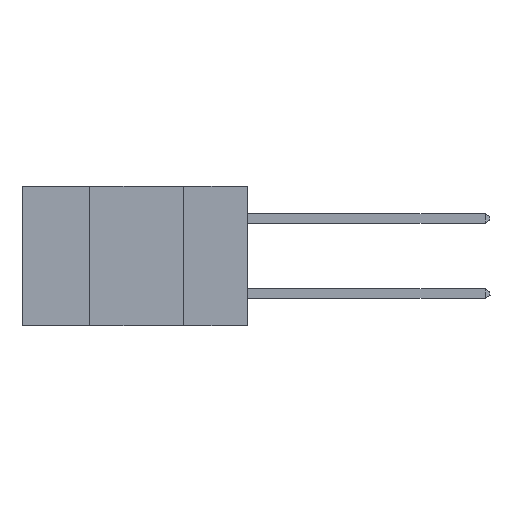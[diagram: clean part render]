
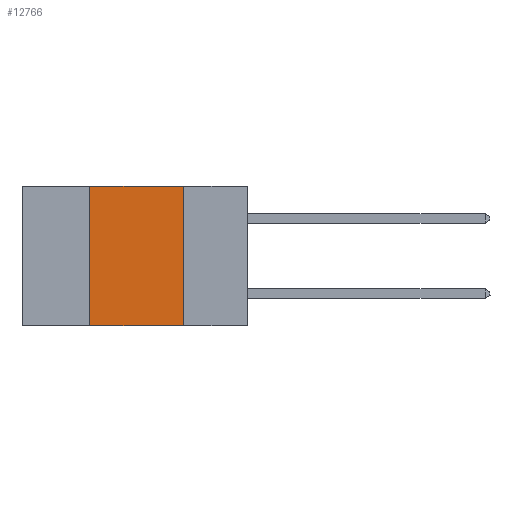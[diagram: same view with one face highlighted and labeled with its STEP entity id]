
A CAD part, left-side view. The second image highlights one B-rep face of the part: STEP entity #12766.
In plain terms, the highlighted planar face has unit normal (-1, 0, 0).
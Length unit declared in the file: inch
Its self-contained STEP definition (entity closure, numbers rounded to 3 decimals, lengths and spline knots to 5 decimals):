
#288 = EDGE_CURVE ( 'NONE', #16798, #23068, #29079, .T. ) ;
#878 = LINE ( 'NONE', #9492, #11123 ) ;
#1423 = CARTESIAN_POINT ( 'NONE',  ( 0., 0.42, 0. ) ) ;
#1833 = DIRECTION ( 'NONE',  ( 0., 0., -1. ) ) ;
#1933 = DIRECTION ( 'NONE',  ( 1., 0., 0. ) ) ;
#2817 = VECTOR ( 'NONE', #6527, 39.37008 ) ;
#5611 = DIRECTION ( 'NONE',  ( 0., -1., 0. ) ) ;
#6152 = VECTOR ( 'NONE', #5611, 39.37008 ) ;
#6527 = DIRECTION ( 'NONE',  ( 0., -1., 0. ) ) ;
#8866 = CARTESIAN_POINT ( 'NONE',  ( 0., 0.6, 0. ) ) ;
#8895 = EDGE_CURVE ( 'NONE', #28290, #23068, #17753, .T. ) ;
#9492 = CARTESIAN_POINT ( 'NONE',  ( 0., 0.42, 0. ) ) ;
#11123 = VECTOR ( 'NONE', #16550, 39.37008 ) ;
#11801 = ORIENTED_EDGE ( 'NONE', *, *, #12406, .F. ) ;
#12406 = EDGE_CURVE ( 'NONE', #28290, #13880, #878, .T. ) ;
#12438 = EDGE_CURVE ( 'NONE', #13880, #16798, #18273, .T. ) ;
#12471 = CARTESIAN_POINT ( 'NONE',  ( 0., 0.6, 0. ) ) ;
#12766 = ADVANCED_FACE ( 'NONE', ( #17528 ), #22303, .F. ) ;
#13751 = CARTESIAN_POINT ( 'NONE',  ( 0., 0.17, 0. ) ) ;
#13880 = VERTEX_POINT ( 'NONE', #1423 ) ;
#14284 = CARTESIAN_POINT ( 'NONE',  ( 0., 0.17, 0. ) ) ;
#14388 = ORIENTED_EDGE ( 'NONE', *, *, #288, .F. ) ;
#16550 = DIRECTION ( 'NONE',  ( 0., 0., 1. ) ) ;
#16798 = VERTEX_POINT ( 'NONE', #13751 ) ;
#17416 = ORIENTED_EDGE ( 'NONE', *, *, #8895, .T. ) ;
#17528 = FACE_OUTER_BOUND ( 'NONE', #23466, .T. ) ;
#17753 = LINE ( 'NONE', #29027, #2817 ) ;
#18273 = LINE ( 'NONE', #12471, #6152 ) ;
#19690 = CARTESIAN_POINT ( 'NONE',  ( 0., 0.17, -0.37 ) ) ;
#19898 = CARTESIAN_POINT ( 'NONE',  ( 0., 0.42, -0.37 ) ) ;
#22303 = PLANE ( 'NONE',  #25338 ) ;
#23068 = VERTEX_POINT ( 'NONE', #19690 ) ;
#23466 = EDGE_LOOP ( 'NONE', ( #14388, #27399, #11801, #17416 ) ) ;
#25338 = AXIS2_PLACEMENT_3D ( 'NONE', #8866, #1933, #1833 ) ;
#25951 = DIRECTION ( 'NONE',  ( 0., 0., -1. ) ) ;
#26256 = VECTOR ( 'NONE', #25951, 39.37008 ) ;
#27399 = ORIENTED_EDGE ( 'NONE', *, *, #12438, .F. ) ;
#28290 = VERTEX_POINT ( 'NONE', #19898 ) ;
#29027 = CARTESIAN_POINT ( 'NONE',  ( 0., 0.6, -0.37 ) ) ;
#29079 = LINE ( 'NONE', #14284, #26256 ) ;
